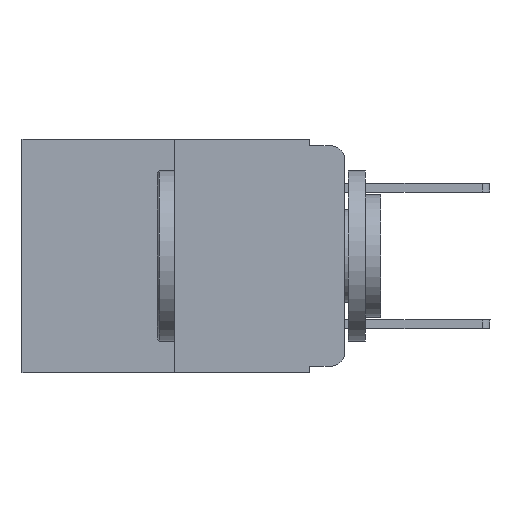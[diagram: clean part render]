
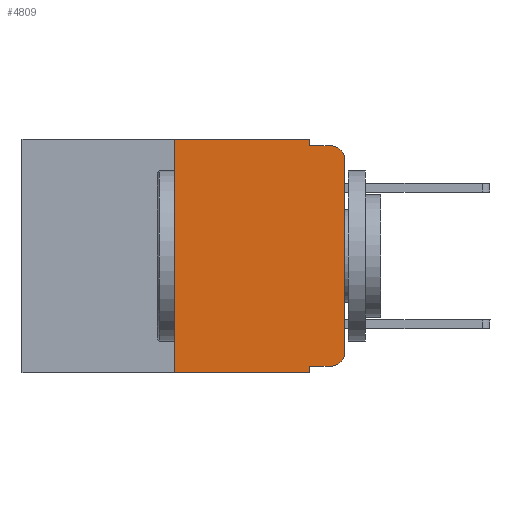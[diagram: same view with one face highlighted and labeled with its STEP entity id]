
A CAD part, left-side view. The second image highlights one B-rep face of the part: STEP entity #4809.
In plain terms, the highlighted planar face has unit normal (-1, 0, 0).
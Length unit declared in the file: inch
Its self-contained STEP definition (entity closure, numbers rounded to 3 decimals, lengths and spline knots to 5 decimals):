
#4 = CARTESIAN_POINT ( 'NONE',  ( 0., 0.051, -0.01 ) ) ;
#213 = CARTESIAN_POINT ( 'NONE',  ( 0., 0., -0.313 ) ) ;
#807 = ORIENTED_EDGE ( 'NONE', *, *, #17773, .F. ) ;
#830 = CARTESIAN_POINT ( 'NONE',  ( 0., 0.02, -0.01 ) ) ;
#964 = AXIS2_PLACEMENT_3D ( 'NONE', #5721, #19026, #5871 ) ;
#1162 = EDGE_LOOP ( 'NONE', ( #2599, #14359, #807, #9552, #13834, #6973, #13746, #7535, #4985, #14436 ) ) ;
#1731 = CARTESIAN_POINT ( 'NONE',  ( 0., 0.473, -0.343 ) ) ;
#1807 = CARTESIAN_POINT ( 'NONE',  ( 0., 0.051, -0.343 ) ) ;
#1868 = VECTOR ( 'NONE', #8655, 39.37008 ) ;
#2274 = FACE_OUTER_BOUND ( 'NONE', #1162, .T. ) ;
#2453 = EDGE_CURVE ( 'NONE', #12528, #9981, #21403, .T. ) ;
#2599 = ORIENTED_EDGE ( 'NONE', *, *, #16561, .T. ) ;
#2634 = CARTESIAN_POINT ( 'NONE',  ( 0., 0.051, 0. ) ) ;
#3043 = VERTEX_POINT ( 'NONE', #13981 ) ;
#3188 = AXIS2_PLACEMENT_3D ( 'NONE', #4840, #6445, #18137 ) ;
#3384 = CARTESIAN_POINT ( 'NONE',  ( 0., 0.25, -0.343 ) ) ;
#3651 = CARTESIAN_POINT ( 'NONE',  ( 0., 0.051, -0.01 ) ) ;
#3778 = VECTOR ( 'NONE', #3889, 39.37008 ) ;
#3889 = DIRECTION ( 'NONE',  ( 0., -1., 0. ) ) ;
#3934 = LINE ( 'NONE', #1731, #1868 ) ;
#4018 = LINE ( 'NONE', #3651, #13159 ) ;
#4065 = PLANE ( 'NONE',  #13191 ) ;
#4187 = CARTESIAN_POINT ( 'NONE',  ( 0., 0.25, 0. ) ) ;
#4274 = CARTESIAN_POINT ( 'NONE',  ( 0., 0.051, -0.333 ) ) ;
#4759 = DIRECTION ( 'NONE',  ( 0., -1., 0. ) ) ;
#4809 = ADVANCED_FACE ( 'NONE', ( #2274 ), #4065, .F. ) ;
#4840 = CARTESIAN_POINT ( 'NONE',  ( 0., 0.02, -0.313 ) ) ;
#4985 = ORIENTED_EDGE ( 'NONE', *, *, #2453, .T. ) ;
#5054 = CARTESIAN_POINT ( 'NONE',  ( 0., 0.051, 0. ) ) ;
#5277 = DIRECTION ( 'NONE',  ( 0., -1., 0. ) ) ;
#5404 = EDGE_CURVE ( 'NONE', #20681, #18621, #21258, .T. ) ;
#5689 = CARTESIAN_POINT ( 'NONE',  ( 0., 0.473, 0. ) ) ;
#5721 = CARTESIAN_POINT ( 'NONE',  ( 0., 0.02, -0.03 ) ) ;
#5871 = DIRECTION ( 'NONE',  ( 0., 0., -1. ) ) ;
#6300 = EDGE_CURVE ( 'NONE', #16780, #19551, #16534, .T. ) ;
#6445 = DIRECTION ( 'NONE',  ( -1., 0., 0. ) ) ;
#6973 = ORIENTED_EDGE ( 'NONE', *, *, #5404, .F. ) ;
#7257 = EDGE_CURVE ( 'NONE', #12528, #18516, #17697, .T. ) ;
#7404 = DIRECTION ( 'NONE',  ( 1., 0., 0. ) ) ;
#7535 = ORIENTED_EDGE ( 'NONE', *, *, #7257, .F. ) ;
#7769 = VERTEX_POINT ( 'NONE', #4 ) ;
#8655 = DIRECTION ( 'NONE',  ( 0., -1., 0. ) ) ;
#9334 = DIRECTION ( 'NONE',  ( 0., 0., 1. ) ) ;
#9552 = ORIENTED_EDGE ( 'NONE', *, *, #19709, .F. ) ;
#9681 = EDGE_CURVE ( 'NONE', #18621, #3043, #13179, .T. ) ;
#9754 = VECTOR ( 'NONE', #9334, 39.37008 ) ;
#9981 = VERTEX_POINT ( 'NONE', #12758 ) ;
#11092 = DIRECTION ( 'NONE',  ( 0., 0., 1. ) ) ;
#12294 = EDGE_CURVE ( 'NONE', #20681, #18516, #3934, .T. ) ;
#12321 = CARTESIAN_POINT ( 'NONE',  ( 0., 0.051, -0.333 ) ) ;
#12524 = VECTOR ( 'NONE', #4759, 39.37008 ) ;
#12528 = VERTEX_POINT ( 'NONE', #12321 ) ;
#12758 = CARTESIAN_POINT ( 'NONE',  ( 0., 0.02, -0.333 ) ) ;
#13022 = VECTOR ( 'NONE', #18416, 39.37008 ) ;
#13159 = VECTOR ( 'NONE', #5277, 39.37008 ) ;
#13179 = LINE ( 'NONE', #15483, #3778 ) ;
#13191 = AXIS2_PLACEMENT_3D ( 'NONE', #5689, #7404, #19068 ) ;
#13467 = LINE ( 'NONE', #19262, #16597 ) ;
#13746 = ORIENTED_EDGE ( 'NONE', *, *, #12294, .T. ) ;
#13834 = ORIENTED_EDGE ( 'NONE', *, *, #9681, .F. ) ;
#13854 = VECTOR ( 'NONE', #17621, 39.37008 ) ;
#13981 = CARTESIAN_POINT ( 'NONE',  ( 0., 0.051, 0. ) ) ;
#14359 = ORIENTED_EDGE ( 'NONE', *, *, #6300, .T. ) ;
#14436 = ORIENTED_EDGE ( 'NONE', *, *, #16273, .T. ) ;
#14906 = LINE ( 'NONE', #2634, #13854 ) ;
#15483 = CARTESIAN_POINT ( 'NONE',  ( 0., 0.473, 0. ) ) ;
#16273 = EDGE_CURVE ( 'NONE', #9981, #20066, #17915, .T. ) ;
#16534 = CIRCLE ( 'NONE', #964, 0.02 ) ;
#16561 = EDGE_CURVE ( 'NONE', #20066, #16780, #13467, .T. ) ;
#16597 = VECTOR ( 'NONE', #11092, 39.37008 ) ;
#16780 = VERTEX_POINT ( 'NONE', #17961 ) ;
#17621 = DIRECTION ( 'NONE',  ( 0., 0., -1. ) ) ;
#17697 = LINE ( 'NONE', #5054, #13022 ) ;
#17773 = EDGE_CURVE ( 'NONE', #7769, #19551, #4018, .T. ) ;
#17915 = CIRCLE ( 'NONE', #3188, 0.02 ) ;
#17961 = CARTESIAN_POINT ( 'NONE',  ( 0., 0., -0.03 ) ) ;
#18137 = DIRECTION ( 'NONE',  ( 0., 0., -1. ) ) ;
#18416 = DIRECTION ( 'NONE',  ( 0., 0., -1. ) ) ;
#18516 = VERTEX_POINT ( 'NONE', #1807 ) ;
#18621 = VERTEX_POINT ( 'NONE', #20359 ) ;
#19026 = DIRECTION ( 'NONE',  ( -1., 0., 0. ) ) ;
#19068 = DIRECTION ( 'NONE',  ( 0., 0., -1. ) ) ;
#19262 = CARTESIAN_POINT ( 'NONE',  ( 0., 0., 0. ) ) ;
#19551 = VERTEX_POINT ( 'NONE', #830 ) ;
#19709 = EDGE_CURVE ( 'NONE', #3043, #7769, #14906, .T. ) ;
#20066 = VERTEX_POINT ( 'NONE', #213 ) ;
#20359 = CARTESIAN_POINT ( 'NONE',  ( 0., 0.25, 0. ) ) ;
#20681 = VERTEX_POINT ( 'NONE', #3384 ) ;
#21258 = LINE ( 'NONE', #4187, #9754 ) ;
#21403 = LINE ( 'NONE', #4274, #12524 ) ;
